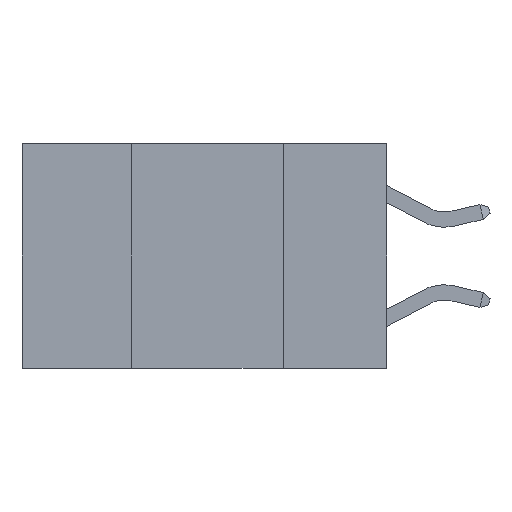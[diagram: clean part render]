
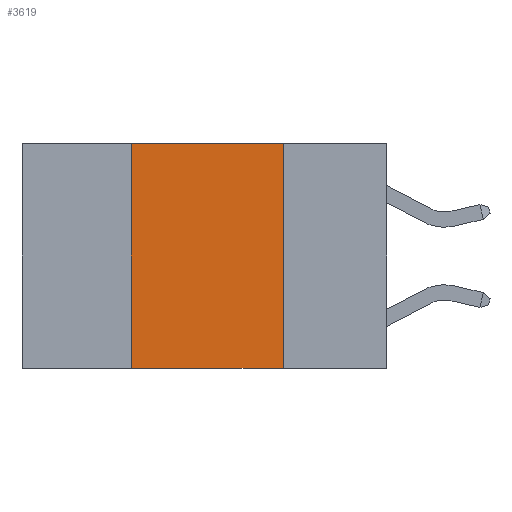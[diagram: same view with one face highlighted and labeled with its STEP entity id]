
A CAD part, left-side view. The second image highlights one B-rep face of the part: STEP entity #3619.
In plain terms, the highlighted planar face has unit normal (-1, 0, 0).
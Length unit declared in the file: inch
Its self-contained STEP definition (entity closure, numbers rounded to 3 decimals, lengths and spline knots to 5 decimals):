
#333 = DIRECTION ( 'NONE',  ( 0., -1., 0. ) ) ;
#380 = ORIENTED_EDGE ( 'NONE', *, *, #4438, .F. ) ;
#386 = ORIENTED_EDGE ( 'NONE', *, *, #6151, .F. ) ;
#529 = PLANE ( 'NONE',  #4483 ) ;
#1027 = VERTEX_POINT ( 'NONE', #10009 ) ;
#1082 = VECTOR ( 'NONE', #8468, 39.37008 ) ;
#1910 = LINE ( 'NONE', #13657, #1082 ) ;
#2018 = EDGE_CURVE ( 'NONE', #7726, #1027, #8694, .T. ) ;
#2043 = EDGE_LOOP ( 'NONE', ( #380, #386, #7761, #12389 ) ) ;
#2375 = VERTEX_POINT ( 'NONE', #14028 ) ;
#3389 = VECTOR ( 'NONE', #333, 39.37008 ) ;
#3552 = CARTESIAN_POINT ( 'NONE',  ( 0., 0.6, 0. ) ) ;
#3619 = ADVANCED_FACE ( 'NONE', ( #12120 ), #529, .F. ) ;
#4438 = EDGE_CURVE ( 'NONE', #12256, #2375, #1910, .T. ) ;
#4483 = AXIS2_PLACEMENT_3D ( 'NONE', #13395, #5736, #6838 ) ;
#5499 = EDGE_CURVE ( 'NONE', #7726, #2375, #12016, .T. ) ;
#5557 = VECTOR ( 'NONE', #10061, 39.37008 ) ;
#5736 = DIRECTION ( 'NONE',  ( 1., 0., 0. ) ) ;
#6151 = EDGE_CURVE ( 'NONE', #1027, #12256, #12745, .T. ) ;
#6493 = VECTOR ( 'NONE', #8478, 39.37008 ) ;
#6838 = DIRECTION ( 'NONE',  ( 0., 0., -1. ) ) ;
#7726 = VERTEX_POINT ( 'NONE', #15309 ) ;
#7761 = ORIENTED_EDGE ( 'NONE', *, *, #2018, .F. ) ;
#8468 = DIRECTION ( 'NONE',  ( 0., 0., -1. ) ) ;
#8478 = DIRECTION ( 'NONE',  ( 0., -1., 0. ) ) ;
#8694 = LINE ( 'NONE', #8860, #5557 ) ;
#8860 = CARTESIAN_POINT ( 'NONE',  ( 0., 0.42, 0. ) ) ;
#10009 = CARTESIAN_POINT ( 'NONE',  ( 0., 0.42, 0. ) ) ;
#10061 = DIRECTION ( 'NONE',  ( 0., 0., 1. ) ) ;
#12016 = LINE ( 'NONE', #12104, #3389 ) ;
#12104 = CARTESIAN_POINT ( 'NONE',  ( 0., 0.6, -0.37 ) ) ;
#12120 = FACE_OUTER_BOUND ( 'NONE', #2043, .T. ) ;
#12256 = VERTEX_POINT ( 'NONE', #13207 ) ;
#12389 = ORIENTED_EDGE ( 'NONE', *, *, #5499, .T. ) ;
#12745 = LINE ( 'NONE', #3552, #6493 ) ;
#13207 = CARTESIAN_POINT ( 'NONE',  ( 0., 0.17, 0. ) ) ;
#13395 = CARTESIAN_POINT ( 'NONE',  ( 0., 0.6, 0. ) ) ;
#13657 = CARTESIAN_POINT ( 'NONE',  ( 0., 0.17, 0. ) ) ;
#14028 = CARTESIAN_POINT ( 'NONE',  ( 0., 0.17, -0.37 ) ) ;
#15309 = CARTESIAN_POINT ( 'NONE',  ( 0., 0.42, -0.37 ) ) ;
